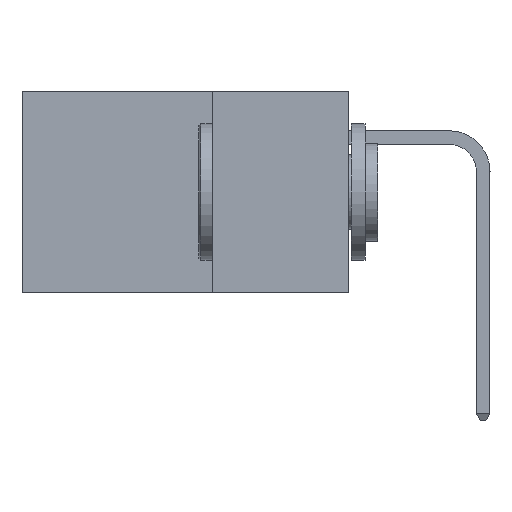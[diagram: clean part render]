
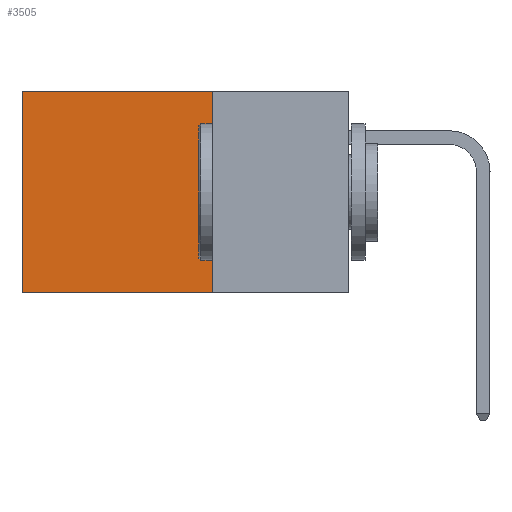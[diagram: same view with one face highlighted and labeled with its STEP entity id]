
A CAD part, left-side view. The second image highlights one B-rep face of the part: STEP entity #3505.
In plain terms, the highlighted planar face has unit normal (-1, 0, 0).
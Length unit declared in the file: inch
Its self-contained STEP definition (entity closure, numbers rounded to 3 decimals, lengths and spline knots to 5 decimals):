
#2185 = VERTEX_POINT ( 'NONE', #33214 ) ;
#2509 = EDGE_CURVE ( 'NONE', #28393, #15687, #31599, .T. ) ;
#3505 = ADVANCED_FACE ( 'NONE', ( #24180 ), #36674, .F. ) ;
#4584 = ORIENTED_EDGE ( 'NONE', *, *, #36671, .F. ) ;
#4997 = CARTESIAN_POINT ( 'NONE',  ( 0.2875, 0.25, 0. ) ) ;
#9263 = CARTESIAN_POINT ( 'NONE',  ( 0.2875, 0.25, -0.37 ) ) ;
#10257 = DIRECTION ( 'NONE',  ( 1., 0., 0. ) ) ;
#11396 = LINE ( 'NONE', #25551, #18397 ) ;
#13882 = DIRECTION ( 'NONE',  ( 0., 1., 0. ) ) ;
#15687 = VERTEX_POINT ( 'NONE', #25216 ) ;
#16102 = EDGE_CURVE ( 'NONE', #2185, #30503, #28495, .T. ) ;
#17497 = ORIENTED_EDGE ( 'NONE', *, *, #16102, .F. ) ;
#18303 = DIRECTION ( 'NONE',  ( 0., 1., 0. ) ) ;
#18397 = VECTOR ( 'NONE', #37087, 39.37008 ) ;
#19216 = EDGE_LOOP ( 'NONE', ( #35432, #17497, #4584, #28540 ) ) ;
#19897 = CARTESIAN_POINT ( 'NONE',  ( 0.2875, 0.25, 0. ) ) ;
#22018 = CARTESIAN_POINT ( 'NONE',  ( 0.2875, 0.25, 0. ) ) ;
#23308 = LINE ( 'NONE', #34413, #28346 ) ;
#24180 = FACE_OUTER_BOUND ( 'NONE', #19216, .T. ) ;
#25216 = CARTESIAN_POINT ( 'NONE',  ( 0.2875, 0.6, 0. ) ) ;
#25551 = CARTESIAN_POINT ( 'NONE',  ( 0.2875, 0.6, 0. ) ) ;
#25655 = DIRECTION ( 'NONE',  ( 0., 0., -1. ) ) ;
#27596 = VECTOR ( 'NONE', #18303, 39.37008 ) ;
#28346 = VECTOR ( 'NONE', #25655, 39.37008 ) ;
#28393 = VERTEX_POINT ( 'NONE', #4997 ) ;
#28495 = LINE ( 'NONE', #9263, #27596 ) ;
#28540 = ORIENTED_EDGE ( 'NONE', *, *, #2509, .T. ) ;
#28960 = CARTESIAN_POINT ( 'NONE',  ( 0.2875, 0.6, -0.37 ) ) ;
#30503 = VERTEX_POINT ( 'NONE', #28960 ) ;
#30661 = VECTOR ( 'NONE', #13882, 39.37008 ) ;
#30999 = DIRECTION ( 'NONE',  ( 0., 0., -1. ) ) ;
#31599 = LINE ( 'NONE', #19897, #30661 ) ;
#33214 = CARTESIAN_POINT ( 'NONE',  ( 0.2875, 0.25, -0.37 ) ) ;
#33496 = AXIS2_PLACEMENT_3D ( 'NONE', #22018, #10257, #30999 ) ;
#33509 = EDGE_CURVE ( 'NONE', #15687, #30503, #11396, .T. ) ;
#34413 = CARTESIAN_POINT ( 'NONE',  ( 0.2875, 0.25, 0. ) ) ;
#35432 = ORIENTED_EDGE ( 'NONE', *, *, #33509, .T. ) ;
#36671 = EDGE_CURVE ( 'NONE', #28393, #2185, #23308, .T. ) ;
#36674 = PLANE ( 'NONE',  #33496 ) ;
#37087 = DIRECTION ( 'NONE',  ( 0., 0., -1. ) ) ;
